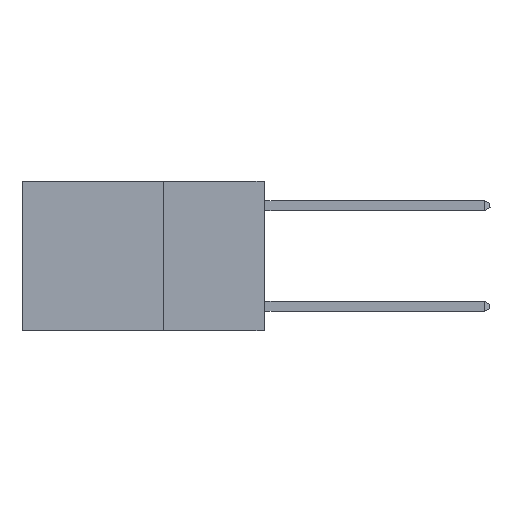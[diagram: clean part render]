
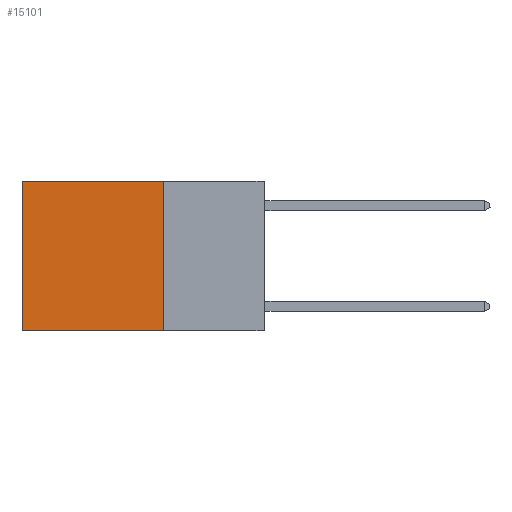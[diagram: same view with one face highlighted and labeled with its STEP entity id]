
A CAD part, left-side view. The second image highlights one B-rep face of the part: STEP entity #15101.
In plain terms, the highlighted planar face has unit normal (-1, 0, 0).
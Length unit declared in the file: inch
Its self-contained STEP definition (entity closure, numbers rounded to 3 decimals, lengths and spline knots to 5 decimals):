
#479 = LINE ( 'NONE', #1182, #7159 ) ;
#1182 = CARTESIAN_POINT ( 'NONE',  ( 0.2625, 0.6, 0. ) ) ;
#1205 = CARTESIAN_POINT ( 'NONE',  ( 0.2625, 0.6, 0. ) ) ;
#1939 = DIRECTION ( 'NONE',  ( 0., 1., 0. ) ) ;
#2540 = FACE_OUTER_BOUND ( 'NONE', #17379, .T. ) ;
#3366 = EDGE_CURVE ( 'NONE', #18307, #10323, #479, .T. ) ;
#4185 = EDGE_CURVE ( 'NONE', #6553, #10323, #9710, .T. ) ;
#6045 = PLANE ( 'NONE',  #15488 ) ;
#6514 = EDGE_CURVE ( 'NONE', #8657, #6553, #11807, .T. ) ;
#6553 = VERTEX_POINT ( 'NONE', #11978 ) ;
#7159 = VECTOR ( 'NONE', #13635, 39.37008 ) ;
#8325 = ORIENTED_EDGE ( 'NONE', *, *, #4185, .F. ) ;
#8327 = VECTOR ( 'NONE', #1939, 39.37008 ) ;
#8657 = VERTEX_POINT ( 'NONE', #11781 ) ;
#8661 = ORIENTED_EDGE ( 'NONE', *, *, #6514, .F. ) ;
#9016 = DIRECTION ( 'NONE',  ( 0., 1., 0. ) ) ;
#9710 = LINE ( 'NONE', #15235, #17034 ) ;
#9777 = LINE ( 'NONE', #11371, #8327 ) ;
#10323 = VERTEX_POINT ( 'NONE', #17966 ) ;
#10646 = DIRECTION ( 'NONE',  ( 1., 0., 0. ) ) ;
#10768 = CARTESIAN_POINT ( 'NONE',  ( 0.2625, 0.25, 0. ) ) ;
#11371 = CARTESIAN_POINT ( 'NONE',  ( 0.2625, 0.25, 0. ) ) ;
#11781 = CARTESIAN_POINT ( 'NONE',  ( 0.2625, 0.25, 0. ) ) ;
#11807 = LINE ( 'NONE', #13693, #18887 ) ;
#11978 = CARTESIAN_POINT ( 'NONE',  ( 0.2625, 0.25, -0.37 ) ) ;
#12036 = ORIENTED_EDGE ( 'NONE', *, *, #20293, .T. ) ;
#12439 = ORIENTED_EDGE ( 'NONE', *, *, #3366, .T. ) ;
#13635 = DIRECTION ( 'NONE',  ( 0., 0., -1. ) ) ;
#13693 = CARTESIAN_POINT ( 'NONE',  ( 0.2625, 0.25, 0. ) ) ;
#15101 = ADVANCED_FACE ( 'NONE', ( #2540 ), #6045, .F. ) ;
#15235 = CARTESIAN_POINT ( 'NONE',  ( 0.2625, 0.25, -0.37 ) ) ;
#15488 = AXIS2_PLACEMENT_3D ( 'NONE', #10768, #10646, #18703 ) ;
#17034 = VECTOR ( 'NONE', #9016, 39.37008 ) ;
#17379 = EDGE_LOOP ( 'NONE', ( #12439, #8325, #8661, #12036 ) ) ;
#17966 = CARTESIAN_POINT ( 'NONE',  ( 0.2625, 0.6, -0.37 ) ) ;
#18307 = VERTEX_POINT ( 'NONE', #1205 ) ;
#18404 = DIRECTION ( 'NONE',  ( 0., 0., -1. ) ) ;
#18703 = DIRECTION ( 'NONE',  ( 0., 0., -1. ) ) ;
#18887 = VECTOR ( 'NONE', #18404, 39.37008 ) ;
#20293 = EDGE_CURVE ( 'NONE', #8657, #18307, #9777, .T. ) ;
